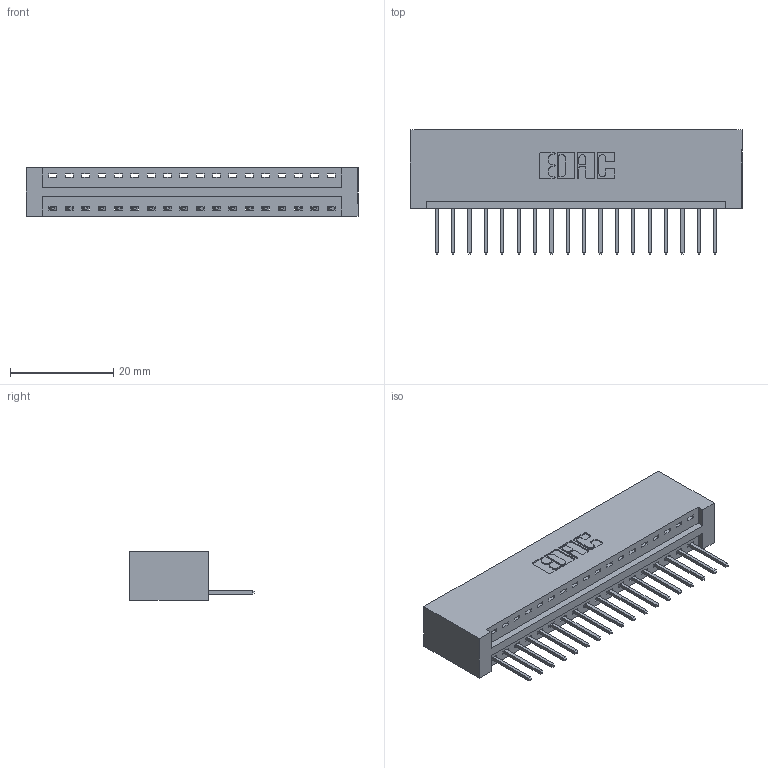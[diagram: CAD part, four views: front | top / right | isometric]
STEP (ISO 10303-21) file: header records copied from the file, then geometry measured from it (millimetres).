
FILE_DESCRIPTION (( 'STEP AP203' ), '1' );
FILE_NAME ('396-018-526-101.STEP', '2019-10-26T19:46:24', ( '' ), ( '' ), 'SwSTEP 2.0', 'SolidWorks 2016', '' );
FILE_SCHEMA (( 'CONFIG_CONTROL_DESIGN' ));
Length unit declared in the file: inch
Products named in the file (3): 396-018-526-101; 346 Part_No Mounting Lugs; 345-292-001_345-293-126
Assembly tree (19 placements, depth 2):
  396-018-526-101
    346 Part_No Mounting Lugs
    345-292-001_345-293-126  x18
Bounding box: 64.39 x 24.13 x 9.4 mm (x, y, z)
Volume: 6533.2 mm3; surface area: 7964.2 mm2
Topology: 19 solids, 19 shells, 1158 faces, 3473 edges, 2290 vertices
Faces by surface type: plane 792, cylinder 366
Entity records: 14143 total; most frequent: CARTESIAN_POINT 2438, ORIENTED_EDGE 2390, DIRECTION 2175, EDGE_CURVE 1195, LINE 999, VECTOR 999, VERTEX_POINT 794, AXIS2_PLACEMENT_3D 588
